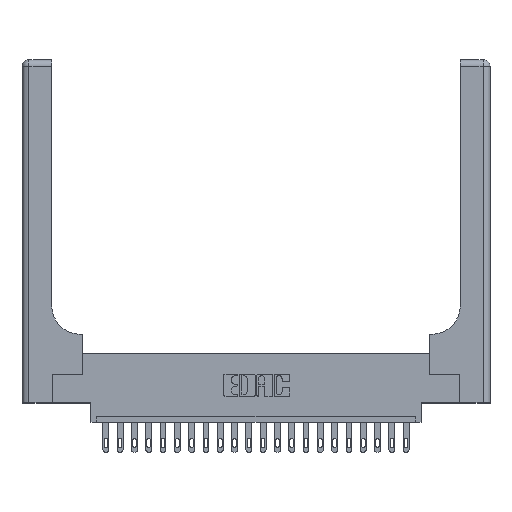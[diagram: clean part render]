
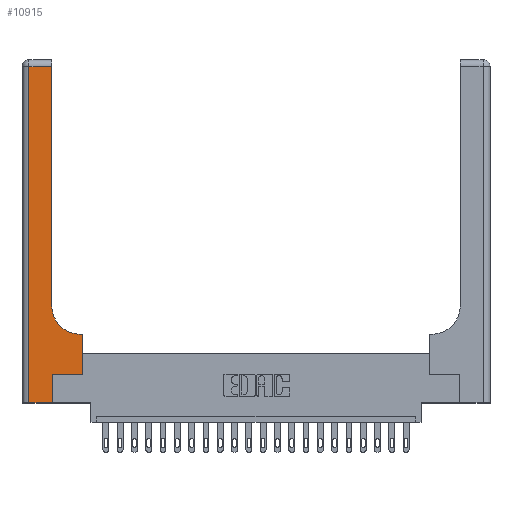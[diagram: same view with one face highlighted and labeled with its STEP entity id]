
A CAD part, top view. The second image highlights one B-rep face of the part: STEP entity #10915.
In plain terms, the highlighted planar face has unit normal (0, 0, 1).
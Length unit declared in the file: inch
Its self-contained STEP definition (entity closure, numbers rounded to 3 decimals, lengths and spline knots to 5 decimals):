
#17 = CARTESIAN_POINT ( 'NONE',  ( 0.528, 0.6, 0.37 ) ) ;
#367 = LINE ( 'NONE', #3202, #10779 ) ;
#372 = DIRECTION ( 'NONE',  ( 0., 1., 0. ) ) ;
#743 = CARTESIAN_POINT ( 'NONE',  ( 0.06, 0., 0.37 ) ) ;
#906 = EDGE_CURVE ( 'NONE', #2404, #6594, #10334, .T. ) ;
#960 = EDGE_CURVE ( 'NONE', #4041, #2404, #9802, .T. ) ;
#1448 = EDGE_CURVE ( 'NONE', #9698, #10696, #10095, .T. ) ;
#1514 = DIRECTION ( 'NONE',  ( -1., 0., 0. ) ) ;
#1935 = ORIENTED_EDGE ( 'NONE', *, *, #960, .T. ) ;
#1990 = ORIENTED_EDGE ( 'NONE', *, *, #3292, .T. ) ;
#2015 = VECTOR ( 'NONE', #10204, 39.37008 ) ;
#2035 = LINE ( 'NONE', #9148, #16178 ) ;
#2095 = DIRECTION ( 'NONE',  ( -1., 0., 0. ) ) ;
#2404 = VERTEX_POINT ( 'NONE', #10136 ) ;
#2564 = CARTESIAN_POINT ( 'NONE',  ( 0.528, 0.25, 0.37 ) ) ;
#2859 = DIRECTION ( 'NONE',  ( 0., 0., -1. ) ) ;
#3202 = CARTESIAN_POINT ( 'NONE',  ( 0.265, 0.25, 0.37 ) ) ;
#3292 = EDGE_CURVE ( 'NONE', #6594, #13180, #2035, .T. ) ;
#4041 = VERTEX_POINT ( 'NONE', #18903 ) ;
#4899 = CARTESIAN_POINT ( 'NONE',  ( 0.51, 0.85, 0.37 ) ) ;
#5154 = ORIENTED_EDGE ( 'NONE', *, *, #5446, .T. ) ;
#5365 = ORIENTED_EDGE ( 'NONE', *, *, #1448, .T. ) ;
#5434 = CARTESIAN_POINT ( 'NONE',  ( 0.265, 0., 0.37 ) ) ;
#5446 = EDGE_CURVE ( 'NONE', #16433, #4041, #10769, .T. ) ;
#6564 = DIRECTION ( 'NONE',  ( 0., 1., 0. ) ) ;
#6594 = VERTEX_POINT ( 'NONE', #21584 ) ;
#6960 = AXIS2_PLACEMENT_3D ( 'NONE', #4899, #8556, #8232 ) ;
#6966 = ORIENTED_EDGE ( 'NONE', *, *, #12678, .T. ) ;
#8232 = DIRECTION ( 'NONE',  ( 1., 0., 0. ) ) ;
#8556 = DIRECTION ( 'NONE',  ( 0., 0., -1. ) ) ;
#9148 = CARTESIAN_POINT ( 'NONE',  ( 0., 2.94, 0.37 ) ) ;
#9225 = CARTESIAN_POINT ( 'NONE',  ( 0.528, 0.25, 0.37 ) ) ;
#9231 = LINE ( 'NONE', #9453, #11738 ) ;
#9351 = DIRECTION ( 'NONE',  ( 0., 1., 0. ) ) ;
#9397 = VECTOR ( 'NONE', #9351, 39.37008 ) ;
#9453 = CARTESIAN_POINT ( 'NONE',  ( 0.06, 3., 0.37 ) ) ;
#9698 = VERTEX_POINT ( 'NONE', #743 ) ;
#9802 = CIRCLE ( 'NONE', #6960, 0.25 ) ;
#10095 = LINE ( 'NONE', #22026, #2015 ) ;
#10136 = CARTESIAN_POINT ( 'NONE',  ( 0.26, 0.85, 0.37 ) ) ;
#10204 = DIRECTION ( 'NONE',  ( 1., 0., 0. ) ) ;
#10289 = LINE ( 'NONE', #15402, #17796 ) ;
#10334 = LINE ( 'NONE', #18582, #20109 ) ;
#10422 = EDGE_CURVE ( 'NONE', #13180, #9698, #9231, .T. ) ;
#10696 = VERTEX_POINT ( 'NONE', #5434 ) ;
#10769 = LINE ( 'NONE', #18910, #18145 ) ;
#10779 = VECTOR ( 'NONE', #14878, 39.37008 ) ;
#10915 = ADVANCED_FACE ( 'NONE', ( #16879 ), #21800, .F. ) ;
#11738 = VECTOR ( 'NONE', #19484, 39.37008 ) ;
#12361 = ORIENTED_EDGE ( 'NONE', *, *, #16000, .T. ) ;
#12678 = EDGE_CURVE ( 'NONE', #10696, #20265, #10289, .T. ) ;
#13180 = VERTEX_POINT ( 'NONE', #14869 ) ;
#14045 = DIRECTION ( 'NONE',  ( -1., 0., 0. ) ) ;
#14869 = CARTESIAN_POINT ( 'NONE',  ( 0.06, 2.94, 0.37 ) ) ;
#14878 = DIRECTION ( 'NONE',  ( 1., 0., 0. ) ) ;
#15402 = CARTESIAN_POINT ( 'NONE',  ( 0.265, 0., 0.37 ) ) ;
#16000 = EDGE_CURVE ( 'NONE', #20265, #21749, #367, .T. ) ;
#16178 = VECTOR ( 'NONE', #14045, 39.37008 ) ;
#16193 = ORIENTED_EDGE ( 'NONE', *, *, #10422, .T. ) ;
#16433 = VERTEX_POINT ( 'NONE', #17 ) ;
#16879 = FACE_OUTER_BOUND ( 'NONE', #17161, .T. ) ;
#17161 = EDGE_LOOP ( 'NONE', ( #19657, #1990, #16193, #5365, #6966, #12361, #19242, #5154, #1935 ) ) ;
#17189 = CARTESIAN_POINT ( 'NONE',  ( 0.265, 0.25, 0.37 ) ) ;
#17796 = VECTOR ( 'NONE', #372, 39.37008 ) ;
#17820 = LINE ( 'NONE', #2564, #9397 ) ;
#18145 = VECTOR ( 'NONE', #2095, 39.37008 ) ;
#18582 = CARTESIAN_POINT ( 'NONE',  ( 0.26, 3., 0.37 ) ) ;
#18903 = CARTESIAN_POINT ( 'NONE',  ( 0.51, 0.6, 0.37 ) ) ;
#18910 = CARTESIAN_POINT ( 'NONE',  ( 0.26, 0.6, 0.37 ) ) ;
#19242 = ORIENTED_EDGE ( 'NONE', *, *, #19899, .T. ) ;
#19484 = DIRECTION ( 'NONE',  ( 0., -1., 0. ) ) ;
#19657 = ORIENTED_EDGE ( 'NONE', *, *, #906, .T. ) ;
#19897 = CARTESIAN_POINT ( 'NONE',  ( 0., 3., 0.37 ) ) ;
#19899 = EDGE_CURVE ( 'NONE', #21749, #16433, #17820, .T. ) ;
#20109 = VECTOR ( 'NONE', #6564, 39.37008 ) ;
#20265 = VERTEX_POINT ( 'NONE', #17189 ) ;
#21364 = AXIS2_PLACEMENT_3D ( 'NONE', #19897, #2859, #1514 ) ;
#21584 = CARTESIAN_POINT ( 'NONE',  ( 0.26, 2.94, 0.37 ) ) ;
#21749 = VERTEX_POINT ( 'NONE', #9225 ) ;
#21800 = PLANE ( 'NONE',  #21364 ) ;
#22026 = CARTESIAN_POINT ( 'NONE',  ( 0., 0., 0.37 ) ) ;
